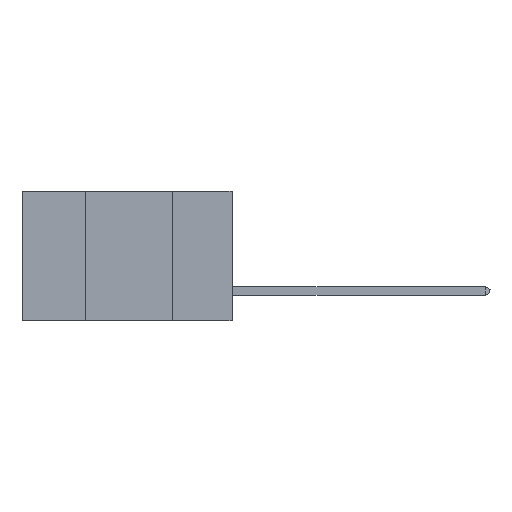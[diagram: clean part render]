
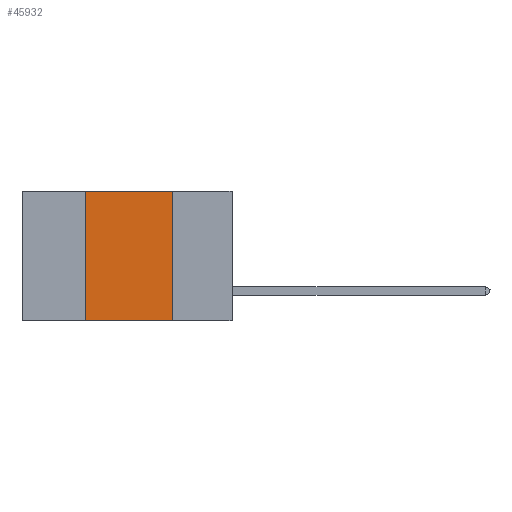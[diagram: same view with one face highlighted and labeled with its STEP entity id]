
A CAD part, left-side view. The second image highlights one B-rep face of the part: STEP entity #45932.
In plain terms, the highlighted planar face has unit normal (-1, 0, 0).
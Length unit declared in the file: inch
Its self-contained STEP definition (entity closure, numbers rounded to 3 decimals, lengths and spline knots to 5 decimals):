
#482 = EDGE_CURVE ( 'NONE', #3982, #2631, #44176, .T. ) ;
#2631 = VERTEX_POINT ( 'NONE', #28636 ) ;
#3226 = CARTESIAN_POINT ( 'NONE',  ( 0., 0.6, 0. ) ) ;
#3711 = VECTOR ( 'NONE', #37818, 39.37008 ) ;
#3811 = EDGE_CURVE ( 'NONE', #38162, #3982, #36278, .T. ) ;
#3911 = DIRECTION ( 'NONE',  ( 0., 0., -1. ) ) ;
#3982 = VERTEX_POINT ( 'NONE', #6884 ) ;
#6884 = CARTESIAN_POINT ( 'NONE',  ( 0., 0.42, 0. ) ) ;
#7506 = EDGE_LOOP ( 'NONE', ( #38321, #43128, #40682, #45010 ) ) ;
#8342 = VECTOR ( 'NONE', #48842, 39.37008 ) ;
#11488 = CARTESIAN_POINT ( 'NONE',  ( 0., 0.17, 0. ) ) ;
#13207 = PLANE ( 'NONE',  #15555 ) ;
#13391 = CARTESIAN_POINT ( 'NONE',  ( 0., 0.6, 0. ) ) ;
#15555 = AXIS2_PLACEMENT_3D ( 'NONE', #13391, #24439, #47316 ) ;
#22424 = VERTEX_POINT ( 'NONE', #44899 ) ;
#22963 = VECTOR ( 'NONE', #3911, 39.37008 ) ;
#24271 = CARTESIAN_POINT ( 'NONE',  ( 0., 0.42, -0.37 ) ) ;
#24439 = DIRECTION ( 'NONE',  ( 1., 0., 0. ) ) ;
#25399 = LINE ( 'NONE', #11488, #22963 ) ;
#28636 = CARTESIAN_POINT ( 'NONE',  ( 0., 0.17, 0. ) ) ;
#31624 = VECTOR ( 'NONE', #48823, 39.37008 ) ;
#34169 = CARTESIAN_POINT ( 'NONE',  ( 0., 0.42, 0. ) ) ;
#36278 = LINE ( 'NONE', #34169, #3711 ) ;
#37818 = DIRECTION ( 'NONE',  ( 0., 0., 1. ) ) ;
#38162 = VERTEX_POINT ( 'NONE', #24271 ) ;
#38321 = ORIENTED_EDGE ( 'NONE', *, *, #46342, .F. ) ;
#40235 = EDGE_CURVE ( 'NONE', #38162, #22424, #41557, .T. ) ;
#40682 = ORIENTED_EDGE ( 'NONE', *, *, #3811, .F. ) ;
#41083 = CARTESIAN_POINT ( 'NONE',  ( 0., 0.6, -0.37 ) ) ;
#41557 = LINE ( 'NONE', #41083, #8342 ) ;
#43128 = ORIENTED_EDGE ( 'NONE', *, *, #482, .F. ) ;
#44176 = LINE ( 'NONE', #3226, #31624 ) ;
#44899 = CARTESIAN_POINT ( 'NONE',  ( 0., 0.17, -0.37 ) ) ;
#45010 = ORIENTED_EDGE ( 'NONE', *, *, #40235, .T. ) ;
#45601 = FACE_OUTER_BOUND ( 'NONE', #7506, .T. ) ;
#45932 = ADVANCED_FACE ( 'NONE', ( #45601 ), #13207, .F. ) ;
#46342 = EDGE_CURVE ( 'NONE', #2631, #22424, #25399, .T. ) ;
#47316 = DIRECTION ( 'NONE',  ( 0., 0., -1. ) ) ;
#48823 = DIRECTION ( 'NONE',  ( 0., -1., 0. ) ) ;
#48842 = DIRECTION ( 'NONE',  ( 0., -1., 0. ) ) ;
